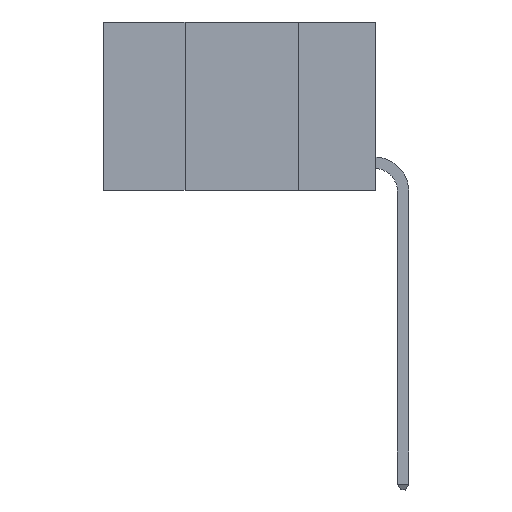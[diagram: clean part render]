
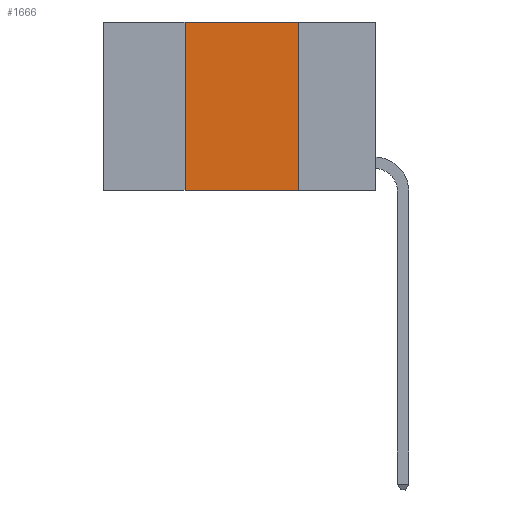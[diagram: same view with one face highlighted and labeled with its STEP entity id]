
A CAD part, left-side view. The second image highlights one B-rep face of the part: STEP entity #1666.
In plain terms, the highlighted planar face has unit normal (-1, 0, 0).
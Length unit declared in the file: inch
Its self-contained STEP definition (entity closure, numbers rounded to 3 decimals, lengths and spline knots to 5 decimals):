
#368 = CARTESIAN_POINT ( 'NONE',  ( 0., 0.42, 0. ) ) ;
#505 = ORIENTED_EDGE ( 'NONE', *, *, #7595, .F. ) ;
#581 = CARTESIAN_POINT ( 'NONE',  ( 0., 0.6, 0. ) ) ;
#960 = DIRECTION ( 'NONE',  ( 0., -1., 0. ) ) ;
#1016 = VECTOR ( 'NONE', #2066, 39.37008 ) ;
#1666 = ADVANCED_FACE ( 'NONE', ( #8509 ), #5358, .F. ) ;
#1675 = EDGE_CURVE ( 'NONE', #7036, #4701, #4470, .T. ) ;
#1984 = DIRECTION ( 'NONE',  ( 1., 0., 0. ) ) ;
#2066 = DIRECTION ( 'NONE',  ( 0., 0., -1. ) ) ;
#2527 = VECTOR ( 'NONE', #960, 39.37008 ) ;
#2828 = ORIENTED_EDGE ( 'NONE', *, *, #7489, .T. ) ;
#3013 = VECTOR ( 'NONE', #8382, 39.37008 ) ;
#3180 = CARTESIAN_POINT ( 'NONE',  ( 0., 0.42, -0.37 ) ) ;
#3272 = LINE ( 'NONE', #5349, #1016 ) ;
#3551 = CARTESIAN_POINT ( 'NONE',  ( 0., 0.17, 0. ) ) ;
#4026 = VERTEX_POINT ( 'NONE', #3180 ) ;
#4470 = LINE ( 'NONE', #581, #2527 ) ;
#4701 = VERTEX_POINT ( 'NONE', #3551 ) ;
#4717 = ORIENTED_EDGE ( 'NONE', *, *, #7566, .F. ) ;
#5004 = CARTESIAN_POINT ( 'NONE',  ( 0., 0.6, 0. ) ) ;
#5148 = CARTESIAN_POINT ( 'NONE',  ( 0., 0.17, -0.37 ) ) ;
#5349 = CARTESIAN_POINT ( 'NONE',  ( 0., 0.17, 0. ) ) ;
#5358 = PLANE ( 'NONE',  #7162 ) ;
#5361 = DIRECTION ( 'NONE',  ( 0., 0., -1. ) ) ;
#5859 = LINE ( 'NONE', #7596, #9624 ) ;
#7036 = VERTEX_POINT ( 'NONE', #7769 ) ;
#7162 = AXIS2_PLACEMENT_3D ( 'NONE', #5004, #1984, #5361 ) ;
#7489 = EDGE_CURVE ( 'NONE', #4026, #9143, #5859, .T. ) ;
#7566 = EDGE_CURVE ( 'NONE', #4701, #9143, #3272, .T. ) ;
#7595 = EDGE_CURVE ( 'NONE', #4026, #7036, #9165, .T. ) ;
#7596 = CARTESIAN_POINT ( 'NONE',  ( 0., 0.6, -0.37 ) ) ;
#7769 = CARTESIAN_POINT ( 'NONE',  ( 0., 0.42, 0. ) ) ;
#8354 = DIRECTION ( 'NONE',  ( 0., -1., 0. ) ) ;
#8382 = DIRECTION ( 'NONE',  ( 0., 0., 1. ) ) ;
#8509 = FACE_OUTER_BOUND ( 'NONE', #9203, .T. ) ;
#8775 = ORIENTED_EDGE ( 'NONE', *, *, #1675, .F. ) ;
#9143 = VERTEX_POINT ( 'NONE', #5148 ) ;
#9165 = LINE ( 'NONE', #368, #3013 ) ;
#9203 = EDGE_LOOP ( 'NONE', ( #4717, #8775, #505, #2828 ) ) ;
#9624 = VECTOR ( 'NONE', #8354, 39.37008 ) ;
